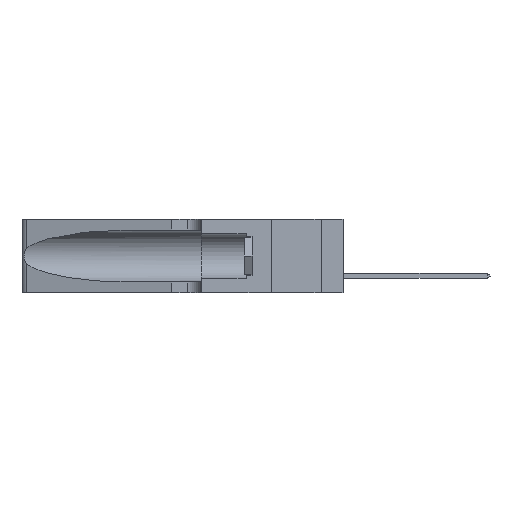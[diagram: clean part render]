
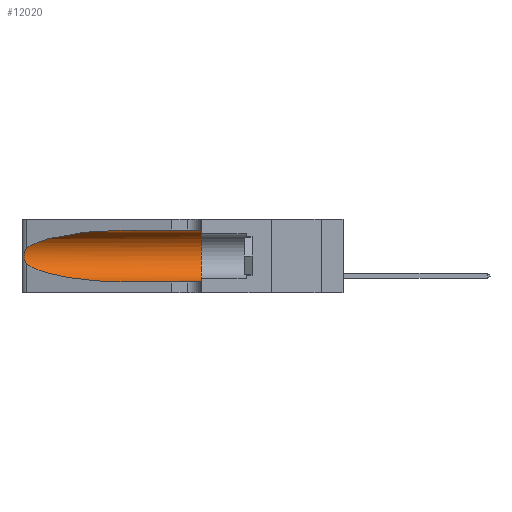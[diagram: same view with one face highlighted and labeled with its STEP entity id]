
A CAD part, left-side view. The second image highlights one B-rep face of the part: STEP entity #12020.
In plain terms, the highlighted cylindrical face has radius 3.308 mm (diameter 6.617 mm), a partial arc.
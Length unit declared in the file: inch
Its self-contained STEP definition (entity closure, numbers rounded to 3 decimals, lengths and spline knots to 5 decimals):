
#311 = CARTESIAN_POINT ( 'NONE',  ( 0.25555, 1.22993, 0.14849 ) ) ;
#1435 = CARTESIAN_POINT ( 'NONE',  ( 0.25487, 1.22718, 0.14631 ) ) ;
#1741 = LINE ( 'NONE', #12964, #16194 ) ;
#1933 = ORIENTED_EDGE ( 'NONE', *, *, #22693, .F. ) ;
#2737 = CARTESIAN_POINT ( 'NONE',  ( 0.25639, 1.23184, 0.21858 ) ) ;
#2829 = CARTESIAN_POINT ( 'NONE',  ( 0.1305, 0.72297, 0.31525 ) ) ;
#3584 = EDGE_CURVE ( 'NONE', #5738, #11010, #21379, .T. ) ;
#3852 = FACE_OUTER_BOUND ( 'NONE', #26536, .T. ) ;
#4249 = ORIENTED_EDGE ( 'NONE', *, *, #5236, .F. ) ;
#5006 = CARTESIAN_POINT ( 'NONE',  ( 0.25555, 1.22994, 0.2215 ) ) ;
#5105 = CARTESIAN_POINT ( 'NONE',  ( 0.25487, 1.22718, 0.14631 ) ) ;
#5236 = EDGE_CURVE ( 'NONE', #27605, #16761, #5753, .T. ) ;
#5524 = CARTESIAN_POINT ( 'NONE',  ( 0.25487, 1.22718, 0.22369 ) ) ;
#5738 = VERTEX_POINT ( 'NONE', #1435 ) ;
#5753 = LINE ( 'NONE', #20939, #16164 ) ;
#6073 = CARTESIAN_POINT ( 'NONE',  ( 0.25487, 1.22718, 0.22369 ) ) ;
#6286 = CARTESIAN_POINT ( 'NONE',  ( 0.18966, 0.96281, 0.05475 ) ) ;
#6351 = EDGE_CURVE ( 'NONE', #27605, #11975, #19646, .T. ) ;
#6372 = DIRECTION ( 'NONE',  ( 0., 0., -1. ) ) ;
#7998 = CARTESIAN_POINT ( 'NONE',  ( 0.18966, 0.96281, 0.31525 ) ) ;
#8858 = CARTESIAN_POINT ( 'NONE',  ( 0.1305, 1.61858, 0.185 ) ) ;
#9669 = CARTESIAN_POINT ( 'NONE',  ( 0.26075, 1.23896, 0.19203 ) ) ;
#10465 = AXIS2_PLACEMENT_3D ( 'NONE', #8858, #22916, #6372 ) ;
#11010 = VERTEX_POINT ( 'NONE', #26846 ) ;
#11559 = DIRECTION ( 'NONE',  ( 0., 1., 0. ) ) ;
#11669 = DIRECTION ( 'NONE',  ( 0., 0., 1. ) ) ;
#11952 = CARTESIAN_POINT ( 'NONE',  ( 0.25789, 1.23486, 0.15765 ) ) ;
#11975 = VERTEX_POINT ( 'NONE', #6073 ) ;
#12020 = ADVANCED_FACE ( 'NONE', ( #3852 ), #25411, .F. ) ;
#12625 = CARTESIAN_POINT ( 'NONE',  ( 0.1305, 0.35, 0.31525 ) ) ;
#12964 = CARTESIAN_POINT ( 'NONE',  ( 0.1305, 1.61858, 0.05475 ) ) ;
#14092 = AXIS2_PLACEMENT_3D ( 'NONE', #18432, #11559, #11669 ) ;
#14547 = CARTESIAN_POINT ( 'NONE',  ( 0.26017, 1.23833, 0.17102 ) ) ;
#15083 = CARTESIAN_POINT ( 'NONE',  ( 0.1305, 0.35, 0.05475 ) ) ;
#16164 = VECTOR ( 'NONE', #30258, 39.37008 ) ;
#16194 = VECTOR ( 'NONE', #22431, 39.37008 ) ;
#16423 = B_SPLINE_CURVE_WITH_KNOTS ( 'NONE', 3,
 ( #26427, #5006, #2737, #23919, #28849, #21605, #9669, #19321, #14547, #21311, #11952, #19224, #311, #5105 ),
 .UNSPECIFIED., .F., .F.,
 ( 4, 2, 2, 2, 2, 2, 4 ),
 ( 0., 0.00027, 0.00053, 0.00107, 0.0016, 0.00187, 0.00214 ),
 .UNSPECIFIED. ) ;
#16457 = VERTEX_POINT ( 'NONE', #15083 ) ;
#16642 = ORIENTED_EDGE ( 'NONE', *, *, #3584, .T. ) ;
#16761 = VERTEX_POINT ( 'NONE', #12625 ) ;
#18222 = CARTESIAN_POINT ( 'NONE',  ( 0.25487, 1.22718, 0.14631 ) ) ;
#18432 = CARTESIAN_POINT ( 'NONE',  ( 0.1305, 0.35, 0.185 ) ) ;
#19224 = CARTESIAN_POINT ( 'NONE',  ( 0.25639, 1.23186, 0.15144 ) ) ;
#19321 = CARTESIAN_POINT ( 'NONE',  ( 0.26075, 1.23896, 0.178 ) ) ;
#19646 =( BOUNDED_CURVE ( )  B_SPLINE_CURVE ( 3, ( #2829, #7998, #19840, #5524 ),
 .UNSPECIFIED., .F., .F. ) 
 B_SPLINE_CURVE_WITH_KNOTS ( ( 4, 4 ),
 ( 1.5708, 2.84003 ),
 .UNSPECIFIED. ) 
 CURVE ( )  GEOMETRIC_REPRESENTATION_ITEM ( )  RATIONAL_B_SPLINE_CURVE ( ( 1., 0.87, 0.87, 1. ) ) 
 REPRESENTATION_ITEM ( '' )  );
#19840 = CARTESIAN_POINT ( 'NONE',  ( 0.2373, 1.15595, 0.28018 ) ) ;
#20634 = CARTESIAN_POINT ( 'NONE',  ( 0.1305, 0.72297, 0.05475 ) ) ;
#20939 = CARTESIAN_POINT ( 'NONE',  ( 0.1305, 1.61858, 0.31525 ) ) ;
#21311 = CARTESIAN_POINT ( 'NONE',  ( 0.25856, 1.23593, 0.16098 ) ) ;
#21379 =( BOUNDED_CURVE ( )  B_SPLINE_CURVE ( 3, ( #18222, #27635, #6286, #20634 ),
 .UNSPECIFIED., .F., .T. ) 
 B_SPLINE_CURVE_WITH_KNOTS ( ( 4, 4 ),
 ( 3.44316, 4.71239 ),
 .UNSPECIFIED. ) 
 CURVE ( )  GEOMETRIC_REPRESENTATION_ITEM ( )  RATIONAL_B_SPLINE_CURVE ( ( 1., 0.87, 0.87, 1. ) ) 
 REPRESENTATION_ITEM ( '' )  );
#21605 = CARTESIAN_POINT ( 'NONE',  ( 0.26018, 1.23835, 0.19895 ) ) ;
#22431 = DIRECTION ( 'NONE',  ( 0., -1., 0. ) ) ;
#22693 = EDGE_CURVE ( 'NONE', #16761, #16457, #25651, .T. ) ;
#22916 = DIRECTION ( 'NONE',  ( 0., -1., 0. ) ) ;
#23080 = CARTESIAN_POINT ( 'NONE',  ( 0.1305, 0.72297, 0.31525 ) ) ;
#23919 = CARTESIAN_POINT ( 'NONE',  ( 0.25787, 1.23484, 0.2124 ) ) ;
#24942 = EDGE_CURVE ( 'NONE', #11010, #16457, #1741, .T. ) ;
#25411 = CYLINDRICAL_SURFACE ( 'NONE', #10465, 0.13025 ) ;
#25651 = CIRCLE ( 'NONE', #14092, 0.13025 ) ;
#26427 = CARTESIAN_POINT ( 'NONE',  ( 0.25487, 1.22718, 0.22369 ) ) ;
#26536 = EDGE_LOOP ( 'NONE', ( #30245, #28908, #16642, #30290, #1933, #4249 ) ) ;
#26846 = CARTESIAN_POINT ( 'NONE',  ( 0.1305, 0.72297, 0.05475 ) ) ;
#27605 = VERTEX_POINT ( 'NONE', #23080 ) ;
#27635 = CARTESIAN_POINT ( 'NONE',  ( 0.2373, 1.15595, 0.08982 ) ) ;
#28849 = CARTESIAN_POINT ( 'NONE',  ( 0.25854, 1.2359, 0.20912 ) ) ;
#28908 = ORIENTED_EDGE ( 'NONE', *, *, #28955, .T. ) ;
#28955 = EDGE_CURVE ( 'NONE', #11975, #5738, #16423, .T. ) ;
#30245 = ORIENTED_EDGE ( 'NONE', *, *, #6351, .T. ) ;
#30258 = DIRECTION ( 'NONE',  ( 0., -1., 0. ) ) ;
#30290 = ORIENTED_EDGE ( 'NONE', *, *, #24942, .T. ) ;
